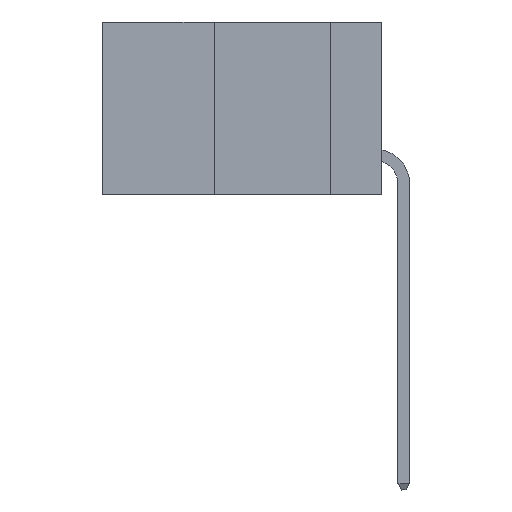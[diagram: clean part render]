
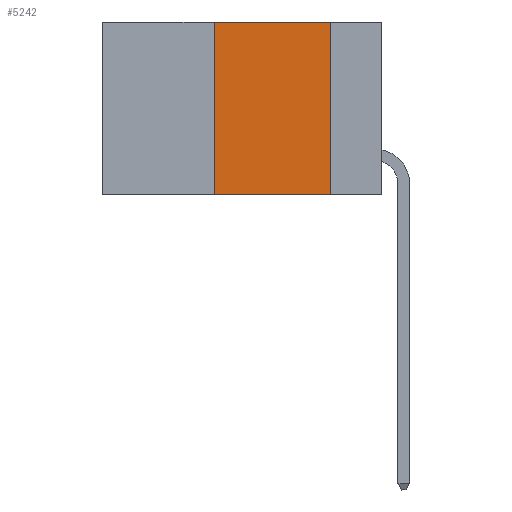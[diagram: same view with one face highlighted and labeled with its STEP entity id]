
A CAD part, left-side view. The second image highlights one B-rep face of the part: STEP entity #5242.
In plain terms, the highlighted planar face has unit normal (-1, 0, 0).
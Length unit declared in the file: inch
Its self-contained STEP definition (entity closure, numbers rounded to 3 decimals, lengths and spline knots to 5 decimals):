
#996 = PLANE ( 'NONE',  #17254 ) ;
#1238 = VECTOR ( 'NONE', #17707, 39.37008 ) ;
#1597 = DIRECTION ( 'NONE',  ( 0., -1., 0. ) ) ;
#2009 = CARTESIAN_POINT ( 'NONE',  ( 0., 0.36, 0. ) ) ;
#3064 = DIRECTION ( 'NONE',  ( 0., 0., -1. ) ) ;
#3402 = DIRECTION ( 'NONE',  ( 0., 0., -1. ) ) ;
#3691 = VECTOR ( 'NONE', #19313, 39.37008 ) ;
#4725 = EDGE_LOOP ( 'NONE', ( #7137, #23739, #25221, #21038 ) ) ;
#5000 = DIRECTION ( 'NONE',  ( 1., 0., 0. ) ) ;
#5061 = CARTESIAN_POINT ( 'NONE',  ( 0., 0.6, -0.37 ) ) ;
#5242 = ADVANCED_FACE ( 'NONE', ( #15333 ), #996, .F. ) ;
#6951 = LINE ( 'NONE', #19804, #1238 ) ;
#7137 = ORIENTED_EDGE ( 'NONE', *, *, #22498, .F. ) ;
#7254 = EDGE_CURVE ( 'NONE', #18381, #12162, #6951, .T. ) ;
#11723 = CARTESIAN_POINT ( 'NONE',  ( 0., 0.6, 0. ) ) ;
#12162 = VERTEX_POINT ( 'NONE', #2009 ) ;
#13215 = EDGE_CURVE ( 'NONE', #18381, #20873, #21427, .T. ) ;
#14938 = CARTESIAN_POINT ( 'NONE',  ( 0., 0.6, 0. ) ) ;
#15333 = FACE_OUTER_BOUND ( 'NONE', #4725, .T. ) ;
#15516 = EDGE_CURVE ( 'NONE', #12162, #22970, #16339, .T. ) ;
#16032 = VECTOR ( 'NONE', #1597, 39.37008 ) ;
#16339 = LINE ( 'NONE', #11723, #16032 ) ;
#17254 = AXIS2_PLACEMENT_3D ( 'NONE', #14938, #5000, #3064 ) ;
#17707 = DIRECTION ( 'NONE',  ( 0., 0., 1. ) ) ;
#18381 = VERTEX_POINT ( 'NONE', #21900 ) ;
#19165 = LINE ( 'NONE', #25851, #26100 ) ;
#19313 = DIRECTION ( 'NONE',  ( 0., -1., 0. ) ) ;
#19804 = CARTESIAN_POINT ( 'NONE',  ( 0., 0.36, 0. ) ) ;
#20873 = VERTEX_POINT ( 'NONE', #25837 ) ;
#21038 = ORIENTED_EDGE ( 'NONE', *, *, #13215, .T. ) ;
#21427 = LINE ( 'NONE', #5061, #3691 ) ;
#21900 = CARTESIAN_POINT ( 'NONE',  ( 0., 0.36, -0.37 ) ) ;
#22498 = EDGE_CURVE ( 'NONE', #22970, #20873, #19165, .T. ) ;
#22970 = VERTEX_POINT ( 'NONE', #25161 ) ;
#23739 = ORIENTED_EDGE ( 'NONE', *, *, #15516, .F. ) ;
#25161 = CARTESIAN_POINT ( 'NONE',  ( 0., 0.11, 0. ) ) ;
#25221 = ORIENTED_EDGE ( 'NONE', *, *, #7254, .F. ) ;
#25837 = CARTESIAN_POINT ( 'NONE',  ( 0., 0.11, -0.37 ) ) ;
#25851 = CARTESIAN_POINT ( 'NONE',  ( 0., 0.11, 0. ) ) ;
#26100 = VECTOR ( 'NONE', #3402, 39.37008 ) ;
